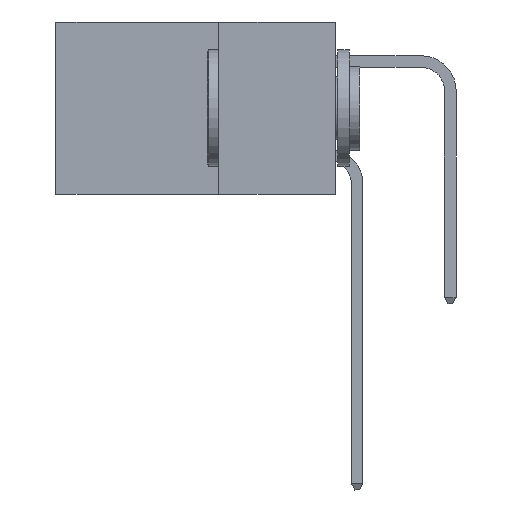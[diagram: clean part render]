
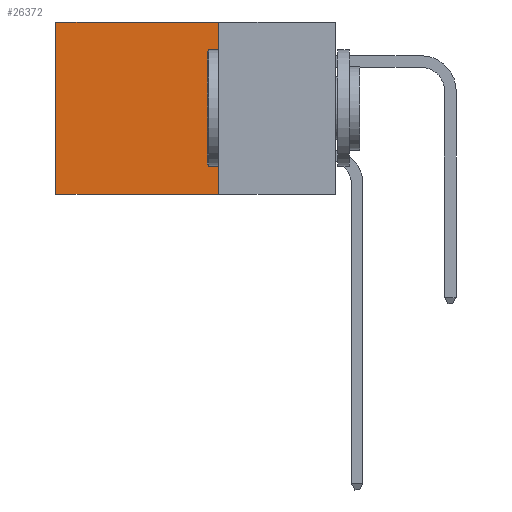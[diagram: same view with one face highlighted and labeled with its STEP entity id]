
A CAD part, left-side view. The second image highlights one B-rep face of the part: STEP entity #26372.
In plain terms, the highlighted planar face has unit normal (-1, 0, 0).
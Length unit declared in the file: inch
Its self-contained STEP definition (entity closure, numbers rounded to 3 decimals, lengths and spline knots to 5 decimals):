
#144 = VERTEX_POINT ( 'NONE', #21851 ) ;
#290 = ORIENTED_EDGE ( 'NONE', *, *, #897, .F. ) ;
#682 = VECTOR ( 'NONE', #8791, 39.37008 ) ;
#897 = EDGE_CURVE ( 'NONE', #144, #1684, #23275, .T. ) ;
#1262 = PLANE ( 'NONE',  #6090 ) ;
#1561 = CARTESIAN_POINT ( 'NONE',  ( 0.2875, 0.25, 0. ) ) ;
#1684 = VERTEX_POINT ( 'NONE', #9073 ) ;
#2627 = VECTOR ( 'NONE', #15847, 39.37008 ) ;
#3506 = CARTESIAN_POINT ( 'NONE',  ( 0.2875, 0.25, -0.37 ) ) ;
#3792 = DIRECTION ( 'NONE',  ( 0., 0., -1. ) ) ;
#4319 = EDGE_CURVE ( 'NONE', #12899, #1684, #23234, .T. ) ;
#5425 = VECTOR ( 'NONE', #30879, 39.37008 ) ;
#5557 = CARTESIAN_POINT ( 'NONE',  ( 0.2875, 0.25, 0. ) ) ;
#6090 = AXIS2_PLACEMENT_3D ( 'NONE', #8480, #25404, #3792 ) ;
#6418 = CARTESIAN_POINT ( 'NONE',  ( 0.2875, 0.25, 0. ) ) ;
#8480 = CARTESIAN_POINT ( 'NONE',  ( 0.2875, 0.25, 0. ) ) ;
#8541 = VECTOR ( 'NONE', #24890, 39.37008 ) ;
#8791 = DIRECTION ( 'NONE',  ( 0., 0., -1. ) ) ;
#9073 = CARTESIAN_POINT ( 'NONE',  ( 0.2875, 0.6, -0.37 ) ) ;
#11297 = EDGE_LOOP ( 'NONE', ( #11927, #290, #28101, #12743 ) ) ;
#11927 = ORIENTED_EDGE ( 'NONE', *, *, #4319, .T. ) ;
#12743 = ORIENTED_EDGE ( 'NONE', *, *, #13487, .T. ) ;
#12899 = VERTEX_POINT ( 'NONE', #30805 ) ;
#13487 = EDGE_CURVE ( 'NONE', #17145, #12899, #17782, .T. ) ;
#15847 = DIRECTION ( 'NONE',  ( 0., 1., 0. ) ) ;
#17145 = VERTEX_POINT ( 'NONE', #5557 ) ;
#17782 = LINE ( 'NONE', #6418, #2627 ) ;
#17789 = FACE_OUTER_BOUND ( 'NONE', #11297, .T. ) ;
#21222 = CARTESIAN_POINT ( 'NONE',  ( 0.2875, 0.6, 0. ) ) ;
#21851 = CARTESIAN_POINT ( 'NONE',  ( 0.2875, 0.25, -0.37 ) ) ;
#21878 = LINE ( 'NONE', #1561, #682 ) ;
#23234 = LINE ( 'NONE', #21222, #5425 ) ;
#23275 = LINE ( 'NONE', #3506, #8541 ) ;
#24890 = DIRECTION ( 'NONE',  ( 0., 1., 0. ) ) ;
#25404 = DIRECTION ( 'NONE',  ( 1., 0., 0. ) ) ;
#26372 = ADVANCED_FACE ( 'NONE', ( #17789 ), #1262, .F. ) ;
#28101 = ORIENTED_EDGE ( 'NONE', *, *, #30335, .F. ) ;
#30335 = EDGE_CURVE ( 'NONE', #17145, #144, #21878, .T. ) ;
#30805 = CARTESIAN_POINT ( 'NONE',  ( 0.2875, 0.6, 0. ) ) ;
#30879 = DIRECTION ( 'NONE',  ( 0., 0., -1. ) ) ;
